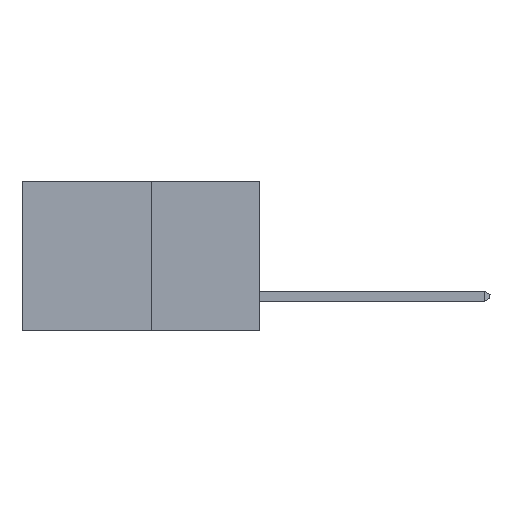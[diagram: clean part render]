
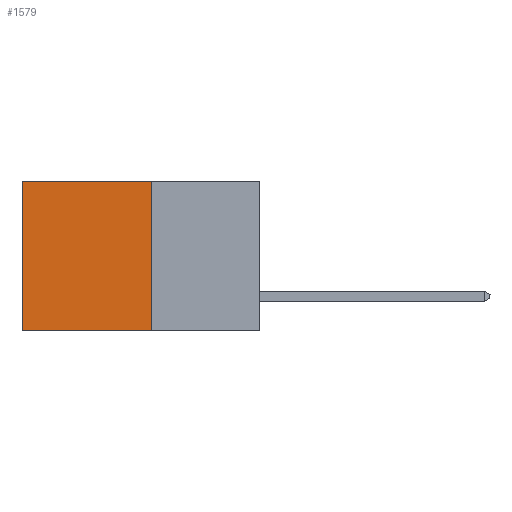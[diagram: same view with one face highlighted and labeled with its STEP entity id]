
A CAD part, left-side view. The second image highlights one B-rep face of the part: STEP entity #1579.
In plain terms, the highlighted planar face has unit normal (-1, 0, 0).
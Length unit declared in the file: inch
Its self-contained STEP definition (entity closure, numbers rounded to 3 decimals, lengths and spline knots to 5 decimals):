
#1579 = ADVANCED_FACE ( 'NONE', ( #20101 ), #21301, .F. ) ;
#1949 = VERTEX_POINT ( 'NONE', #16851 ) ;
#2754 = VECTOR ( 'NONE', #4849, 39.37008 ) ;
#3136 = VERTEX_POINT ( 'NONE', #3353 ) ;
#3353 = CARTESIAN_POINT ( 'NONE',  ( 0.277, 0.27, -0.37 ) ) ;
#3390 = EDGE_LOOP ( 'NONE', ( #4462, #13136, #20583, #21712 ) ) ;
#3800 = LINE ( 'NONE', #17889, #19023 ) ;
#4371 = VECTOR ( 'NONE', #20407, 39.37008 ) ;
#4462 = ORIENTED_EDGE ( 'NONE', *, *, #7799, .T. ) ;
#4747 = VECTOR ( 'NONE', #13312, 39.37008 ) ;
#4849 = DIRECTION ( 'NONE',  ( 0., 0., -1. ) ) ;
#5984 = EDGE_CURVE ( 'NONE', #21191, #3136, #14971, .T. ) ;
#6513 = CARTESIAN_POINT ( 'NONE',  ( 0.277, 0.27, -0.37 ) ) ;
#7799 = EDGE_CURVE ( 'NONE', #1949, #15627, #18630, .T. ) ;
#9304 = CARTESIAN_POINT ( 'NONE',  ( 0.277, 0.27, -0.37 ) ) ;
#10797 = EDGE_CURVE ( 'NONE', #3136, #15627, #20235, .T. ) ;
#11084 = EDGE_CURVE ( 'NONE', #21191, #1949, #3800, .T. ) ;
#12376 = DIRECTION ( 'NONE',  ( 0., 0., -1. ) ) ;
#12411 = DIRECTION ( 'NONE',  ( 1., 0., 0. ) ) ;
#13136 = ORIENTED_EDGE ( 'NONE', *, *, #10797, .F. ) ;
#13312 = DIRECTION ( 'NONE',  ( 0., 1., 0. ) ) ;
#13702 = CARTESIAN_POINT ( 'NONE',  ( 0.277, 0.27, 0. ) ) ;
#14971 = LINE ( 'NONE', #6513, #4371 ) ;
#15627 = VERTEX_POINT ( 'NONE', #22726 ) ;
#16851 = CARTESIAN_POINT ( 'NONE',  ( 0.277, 0.59, 0. ) ) ;
#17889 = CARTESIAN_POINT ( 'NONE',  ( 0.277, 0.27, 0. ) ) ;
#18630 = LINE ( 'NONE', #18755, #2754 ) ;
#18755 = CARTESIAN_POINT ( 'NONE',  ( 0.277, 0.59, -0.37 ) ) ;
#19023 = VECTOR ( 'NONE', #21915, 39.37008 ) ;
#20101 = FACE_OUTER_BOUND ( 'NONE', #3390, .T. ) ;
#20235 = LINE ( 'NONE', #9304, #4747 ) ;
#20407 = DIRECTION ( 'NONE',  ( 0., 0., -1. ) ) ;
#20583 = ORIENTED_EDGE ( 'NONE', *, *, #5984, .F. ) ;
#21132 = CARTESIAN_POINT ( 'NONE',  ( 0.277, 0.27, -0.37 ) ) ;
#21191 = VERTEX_POINT ( 'NONE', #13702 ) ;
#21301 = PLANE ( 'NONE',  #23805 ) ;
#21712 = ORIENTED_EDGE ( 'NONE', *, *, #11084, .T. ) ;
#21915 = DIRECTION ( 'NONE',  ( 0., 1., 0. ) ) ;
#22726 = CARTESIAN_POINT ( 'NONE',  ( 0.277, 0.59, -0.37 ) ) ;
#23805 = AXIS2_PLACEMENT_3D ( 'NONE', #21132, #12411, #12376 ) ;
